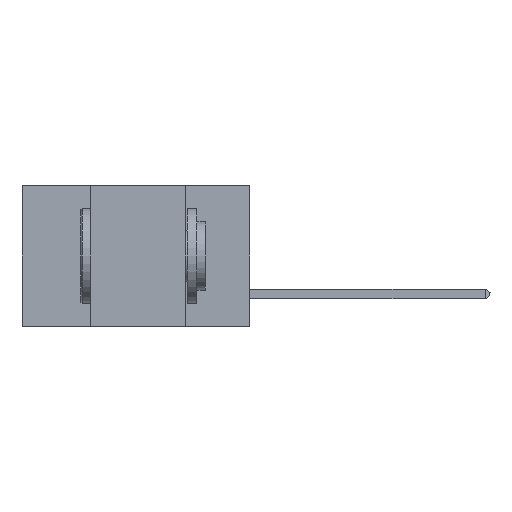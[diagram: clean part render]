
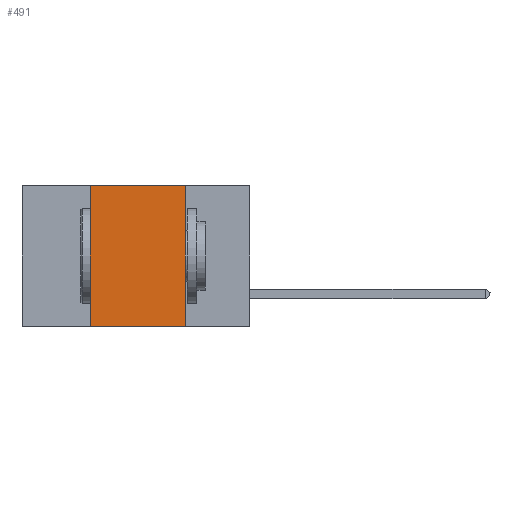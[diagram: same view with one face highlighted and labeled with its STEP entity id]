
A CAD part, left-side view. The second image highlights one B-rep face of the part: STEP entity #491.
In plain terms, the highlighted planar face has unit normal (-1, 0, 0).
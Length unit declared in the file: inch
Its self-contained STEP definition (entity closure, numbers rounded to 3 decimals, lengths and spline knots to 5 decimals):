
#491 = ADVANCED_FACE ( 'NONE', ( #5796 ), #4166, .F. ) ;
#864 = VERTEX_POINT ( 'NONE', #6662 ) ;
#1137 = LINE ( 'NONE', #12826, #11063 ) ;
#1315 = DIRECTION ( 'NONE',  ( 0., 0., -1. ) ) ;
#1719 = ORIENTED_EDGE ( 'NONE', *, *, #4964, .T. ) ;
#1766 = EDGE_CURVE ( 'NONE', #13002, #11213, #16993, .T. ) ;
#2807 = DIRECTION ( 'NONE',  ( 0., 0., -1. ) ) ;
#3881 = EDGE_LOOP ( 'NONE', ( #5954, #18943, #15461, #1719 ) ) ;
#4166 = PLANE ( 'NONE',  #5682 ) ;
#4424 = VERTEX_POINT ( 'NONE', #5981 ) ;
#4713 = EDGE_CURVE ( 'NONE', #864, #4424, #1137, .T. ) ;
#4855 = LINE ( 'NONE', #15488, #11511 ) ;
#4964 = EDGE_CURVE ( 'NONE', #864, #11213, #4855, .T. ) ;
#5682 = AXIS2_PLACEMENT_3D ( 'NONE', #17674, #16069, #1315 ) ;
#5796 = FACE_OUTER_BOUND ( 'NONE', #3881, .T. ) ;
#5954 = ORIENTED_EDGE ( 'NONE', *, *, #1766, .F. ) ;
#5981 = CARTESIAN_POINT ( 'NONE',  ( 0., 0.42, 0. ) ) ;
#6662 = CARTESIAN_POINT ( 'NONE',  ( 0., 0.42, -0.37 ) ) ;
#8723 = CARTESIAN_POINT ( 'NONE',  ( 0., 0.6, 0. ) ) ;
#9360 = CARTESIAN_POINT ( 'NONE',  ( 0., 0.17, 0. ) ) ;
#9415 = EDGE_CURVE ( 'NONE', #4424, #13002, #12842, .T. ) ;
#11063 = VECTOR ( 'NONE', #17294, 39.37008 ) ;
#11213 = VERTEX_POINT ( 'NONE', #14605 ) ;
#11511 = VECTOR ( 'NONE', #12415, 39.37008 ) ;
#12032 = CARTESIAN_POINT ( 'NONE',  ( 0., 0.17, 0. ) ) ;
#12415 = DIRECTION ( 'NONE',  ( 0., -1., 0. ) ) ;
#12826 = CARTESIAN_POINT ( 'NONE',  ( 0., 0.42, 0. ) ) ;
#12842 = LINE ( 'NONE', #8723, #16572 ) ;
#13002 = VERTEX_POINT ( 'NONE', #9360 ) ;
#14605 = CARTESIAN_POINT ( 'NONE',  ( 0., 0.17, -0.37 ) ) ;
#15461 = ORIENTED_EDGE ( 'NONE', *, *, #4713, .F. ) ;
#15488 = CARTESIAN_POINT ( 'NONE',  ( 0., 0.6, -0.37 ) ) ;
#15817 = VECTOR ( 'NONE', #2807, 39.37008 ) ;
#16069 = DIRECTION ( 'NONE',  ( 1., 0., 0. ) ) ;
#16572 = VECTOR ( 'NONE', #17497, 39.37008 ) ;
#16993 = LINE ( 'NONE', #12032, #15817 ) ;
#17294 = DIRECTION ( 'NONE',  ( 0., 0., 1. ) ) ;
#17497 = DIRECTION ( 'NONE',  ( 0., -1., 0. ) ) ;
#17674 = CARTESIAN_POINT ( 'NONE',  ( 0., 0.6, 0. ) ) ;
#18943 = ORIENTED_EDGE ( 'NONE', *, *, #9415, .F. ) ;
